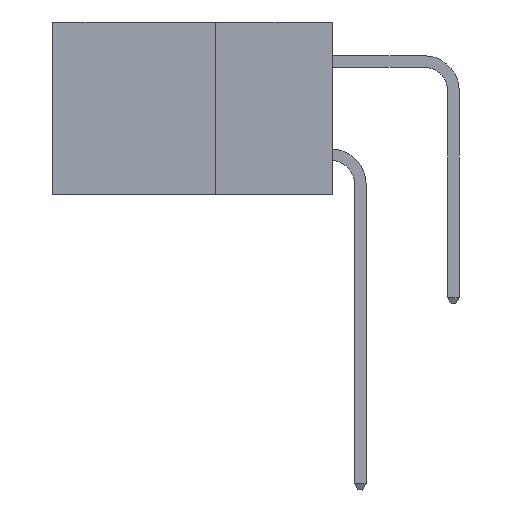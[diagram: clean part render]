
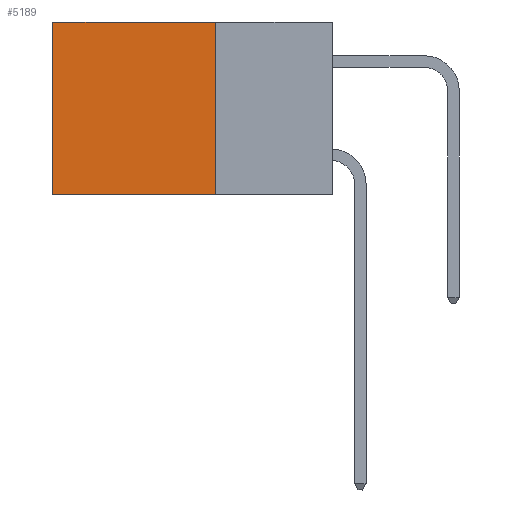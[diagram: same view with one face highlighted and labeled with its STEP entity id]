
A CAD part, left-side view. The second image highlights one B-rep face of the part: STEP entity #5189.
In plain terms, the highlighted planar face has unit normal (-1, 0, 0).
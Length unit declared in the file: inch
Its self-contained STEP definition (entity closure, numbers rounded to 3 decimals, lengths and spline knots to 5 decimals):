
#1542 = EDGE_CURVE ( 'NONE', #5565, #6972, #18031, .T. ) ;
#1625 = CARTESIAN_POINT ( 'NONE',  ( 0.298, 0.25, 0. ) ) ;
#1848 = EDGE_CURVE ( 'NONE', #10768, #6972, #1996, .T. ) ;
#1996 = LINE ( 'NONE', #4376, #4074 ) ;
#2033 = DIRECTION ( 'NONE',  ( 0., 1., 0. ) ) ;
#2256 = AXIS2_PLACEMENT_3D ( 'NONE', #2518, #7032, #13035 ) ;
#2518 = CARTESIAN_POINT ( 'NONE',  ( 0.298, 0.25, 0. ) ) ;
#2628 = DIRECTION ( 'NONE',  ( 0., 1., 0. ) ) ;
#2675 = DIRECTION ( 'NONE',  ( 0., 0., -1. ) ) ;
#4074 = VECTOR ( 'NONE', #2675, 39.37008 ) ;
#4376 = CARTESIAN_POINT ( 'NONE',  ( 0.298, 0.6, 0. ) ) ;
#4614 = EDGE_CURVE ( 'NONE', #15330, #10768, #6519, .T. ) ;
#5189 = ADVANCED_FACE ( 'NONE', ( #17194 ), #11518, .F. ) ;
#5222 = ORIENTED_EDGE ( 'NONE', *, *, #18073, .F. ) ;
#5565 = VERTEX_POINT ( 'NONE', #7080 ) ;
#6519 = LINE ( 'NONE', #9986, #12910 ) ;
#6835 = ORIENTED_EDGE ( 'NONE', *, *, #1848, .T. ) ;
#6972 = VERTEX_POINT ( 'NONE', #18809 ) ;
#7032 = DIRECTION ( 'NONE',  ( 1., 0., 0. ) ) ;
#7080 = CARTESIAN_POINT ( 'NONE',  ( 0.298, 0.25, -0.37 ) ) ;
#7284 = LINE ( 'NONE', #1625, #19346 ) ;
#8044 = CARTESIAN_POINT ( 'NONE',  ( 0.298, 0.25, -0.37 ) ) ;
#8130 = DIRECTION ( 'NONE',  ( 0., 0., -1. ) ) ;
#8330 = CARTESIAN_POINT ( 'NONE',  ( 0.298, 0.25, 0. ) ) ;
#9346 = ORIENTED_EDGE ( 'NONE', *, *, #1542, .F. ) ;
#9986 = CARTESIAN_POINT ( 'NONE',  ( 0.298, 0.25, 0. ) ) ;
#10768 = VERTEX_POINT ( 'NONE', #13248 ) ;
#11518 = PLANE ( 'NONE',  #2256 ) ;
#12910 = VECTOR ( 'NONE', #2628, 39.37008 ) ;
#13035 = DIRECTION ( 'NONE',  ( 0., 0., -1. ) ) ;
#13248 = CARTESIAN_POINT ( 'NONE',  ( 0.298, 0.6, 0. ) ) ;
#13961 = VECTOR ( 'NONE', #2033, 39.37008 ) ;
#15330 = VERTEX_POINT ( 'NONE', #8330 ) ;
#17016 = EDGE_LOOP ( 'NONE', ( #6835, #9346, #5222, #17982 ) ) ;
#17194 = FACE_OUTER_BOUND ( 'NONE', #17016, .T. ) ;
#17982 = ORIENTED_EDGE ( 'NONE', *, *, #4614, .T. ) ;
#18031 = LINE ( 'NONE', #8044, #13961 ) ;
#18073 = EDGE_CURVE ( 'NONE', #15330, #5565, #7284, .T. ) ;
#18809 = CARTESIAN_POINT ( 'NONE',  ( 0.298, 0.6, -0.37 ) ) ;
#19346 = VECTOR ( 'NONE', #8130, 39.37008 ) ;
